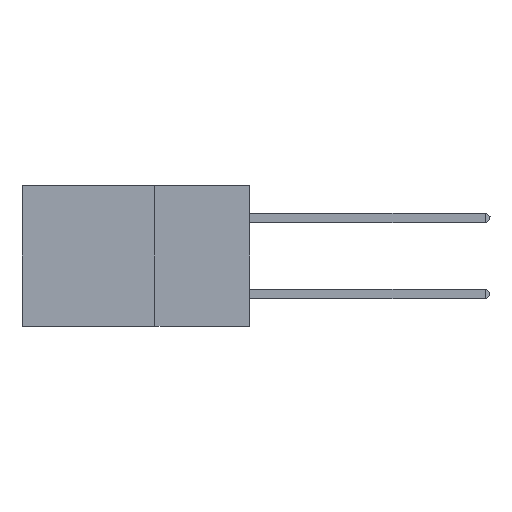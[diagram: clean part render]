
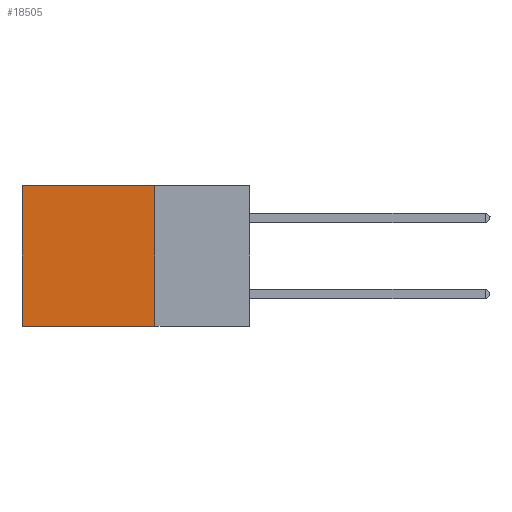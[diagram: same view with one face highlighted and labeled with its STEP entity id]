
A CAD part, left-side view. The second image highlights one B-rep face of the part: STEP entity #18505.
In plain terms, the highlighted planar face has unit normal (-1, 0, 0).
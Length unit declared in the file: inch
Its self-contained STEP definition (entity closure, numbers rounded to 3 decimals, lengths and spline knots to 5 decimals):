
#572 = EDGE_LOOP ( 'NONE', ( #8493, #7127, #1836, #37181 ) ) ;
#1601 = EDGE_CURVE ( 'NONE', #15956, #19620, #3815, .T. ) ;
#1836 = ORIENTED_EDGE ( 'NONE', *, *, #29256, .F. ) ;
#2073 = CARTESIAN_POINT ( 'NONE',  ( 0.2875, 0.25, 0. ) ) ;
#2232 = CARTESIAN_POINT ( 'NONE',  ( 0.2875, 0.25, -0.37 ) ) ;
#2577 = CARTESIAN_POINT ( 'NONE',  ( 0.2875, 0.25, -0.37 ) ) ;
#3815 = LINE ( 'NONE', #10294, #12780 ) ;
#6785 = CARTESIAN_POINT ( 'NONE',  ( 0.2875, 0.6, 0. ) ) ;
#7127 = ORIENTED_EDGE ( 'NONE', *, *, #23716, .F. ) ;
#8493 = ORIENTED_EDGE ( 'NONE', *, *, #38030, .T. ) ;
#10294 = CARTESIAN_POINT ( 'NONE',  ( 0.2875, 0.25, 0. ) ) ;
#10744 = LINE ( 'NONE', #6785, #18243 ) ;
#10781 = CARTESIAN_POINT ( 'NONE',  ( 0.2875, 0.25, 0. ) ) ;
#12740 = DIRECTION ( 'NONE',  ( 1., 0., 0. ) ) ;
#12780 = VECTOR ( 'NONE', #16541, 39.37008 ) ;
#14319 = AXIS2_PLACEMENT_3D ( 'NONE', #22730, #12740, #25470 ) ;
#15857 = FACE_OUTER_BOUND ( 'NONE', #572, .T. ) ;
#15956 = VERTEX_POINT ( 'NONE', #10781 ) ;
#16372 = DIRECTION ( 'NONE',  ( 0., 0., -1. ) ) ;
#16422 = CARTESIAN_POINT ( 'NONE',  ( 0.2875, 0.6, -0.37 ) ) ;
#16541 = DIRECTION ( 'NONE',  ( 0., 1., 0. ) ) ;
#18243 = VECTOR ( 'NONE', #16372, 39.37008 ) ;
#18505 = ADVANCED_FACE ( 'NONE', ( #15857 ), #19393, .F. ) ;
#18908 = LINE ( 'NONE', #2073, #31067 ) ;
#19393 = PLANE ( 'NONE',  #14319 ) ;
#19620 = VERTEX_POINT ( 'NONE', #28266 ) ;
#21427 = LINE ( 'NONE', #2232, #24184 ) ;
#22456 = VERTEX_POINT ( 'NONE', #16422 ) ;
#22730 = CARTESIAN_POINT ( 'NONE',  ( 0.2875, 0.25, 0. ) ) ;
#23716 = EDGE_CURVE ( 'NONE', #32956, #22456, #21427, .T. ) ;
#24184 = VECTOR ( 'NONE', #34153, 39.37008 ) ;
#25470 = DIRECTION ( 'NONE',  ( 0., 0., -1. ) ) ;
#28266 = CARTESIAN_POINT ( 'NONE',  ( 0.2875, 0.6, 0. ) ) ;
#29256 = EDGE_CURVE ( 'NONE', #15956, #32956, #18908, .T. ) ;
#31067 = VECTOR ( 'NONE', #31631, 39.37008 ) ;
#31631 = DIRECTION ( 'NONE',  ( 0., 0., -1. ) ) ;
#32956 = VERTEX_POINT ( 'NONE', #2577 ) ;
#34153 = DIRECTION ( 'NONE',  ( 0., 1., 0. ) ) ;
#37181 = ORIENTED_EDGE ( 'NONE', *, *, #1601, .T. ) ;
#38030 = EDGE_CURVE ( 'NONE', #19620, #22456, #10744, .T. ) ;
